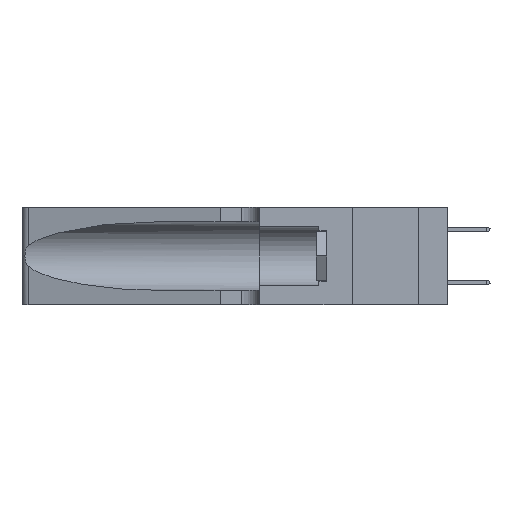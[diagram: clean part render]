
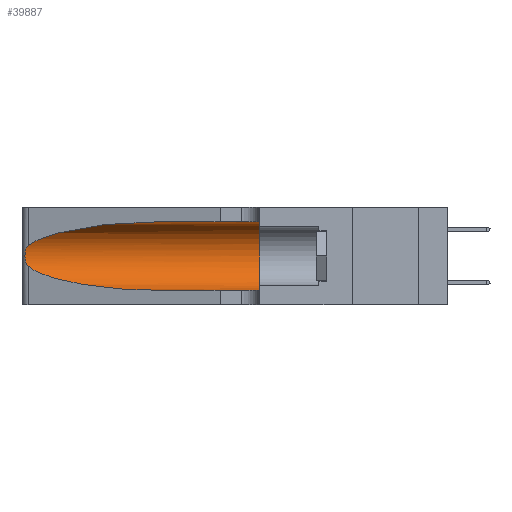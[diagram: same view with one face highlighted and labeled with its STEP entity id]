
A CAD part, left-side view. The second image highlights one B-rep face of the part: STEP entity #39887.
In plain terms, the highlighted cylindrical face has radius 3.308 mm (diameter 6.617 mm), a partial arc.
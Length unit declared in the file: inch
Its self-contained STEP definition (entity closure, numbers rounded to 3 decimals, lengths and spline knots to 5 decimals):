
#478 = CARTESIAN_POINT ( 'NONE',  ( 0.18966, 0.96281, 0.31525 ) ) ;
#2114 = CARTESIAN_POINT ( 'NONE',  ( 0.25487, 1.22718, 0.22369 ) ) ;
#2186 = CYLINDRICAL_SURFACE ( 'NONE', #13376, 0.13025 ) ;
#2251 = CARTESIAN_POINT ( 'NONE',  ( 0.26075, 1.23896, 0.19203 ) ) ;
#3133 = VERTEX_POINT ( 'NONE', #14538 ) ;
#3681 = CARTESIAN_POINT ( 'NONE',  ( 0.2373, 1.15595, 0.28018 ) ) ;
#5518 = CARTESIAN_POINT ( 'NONE',  ( 0.26017, 1.23833, 0.17102 ) ) ;
#5655 = CARTESIAN_POINT ( 'NONE',  ( 0.18966, 0.96281, 0.05475 ) ) ;
#7068 = VECTOR ( 'NONE', #11288, 39.37008 ) ;
#8756 = CARTESIAN_POINT ( 'NONE',  ( 0.25789, 1.23486, 0.15765 ) ) ;
#9062 = DIRECTION ( 'NONE',  ( 0., 1., 0. ) ) ;
#10516 = EDGE_CURVE ( 'NONE', #3133, #27288, #33962, .T. ) ;
#10904 = CARTESIAN_POINT ( 'NONE',  ( 0.1305, 0.35, 0.05475 ) ) ;
#11197 = EDGE_CURVE ( 'NONE', #15068, #31761, #40780, .T. ) ;
#11288 = DIRECTION ( 'NONE',  ( 0., -1., 0. ) ) ;
#11788 = CARTESIAN_POINT ( 'NONE',  ( 0.1305, 0.72297, 0.31525 ) ) ;
#11969 = CARTESIAN_POINT ( 'NONE',  ( 0.25555, 1.22993, 0.14849 ) ) ;
#11972 = CARTESIAN_POINT ( 'NONE',  ( 0.2373, 1.15595, 0.08982 ) ) ;
#12216 = EDGE_CURVE ( 'NONE', #15068, #3133, #19265, .T. ) ;
#12989 = CARTESIAN_POINT ( 'NONE',  ( 0.1305, 0.72297, 0.05475 ) ) ;
#13003 = CARTESIAN_POINT ( 'NONE',  ( 0.1305, 0.35, 0.31525 ) ) ;
#13142 = ORIENTED_EDGE ( 'NONE', *, *, #12216, .T. ) ;
#13376 = AXIS2_PLACEMENT_3D ( 'NONE', #39045, #26362, #20112 ) ;
#13377 = CIRCLE ( 'NONE', #17214, 0.13025 ) ;
#14538 = CARTESIAN_POINT ( 'NONE',  ( 0.25487, 1.22718, 0.22369 ) ) ;
#14853 = DIRECTION ( 'NONE',  ( 0., -1., 0. ) ) ;
#15068 = VERTEX_POINT ( 'NONE', #11788 ) ;
#15341 = ORIENTED_EDGE ( 'NONE', *, *, #11197, .F. ) ;
#15547 = VECTOR ( 'NONE', #14853, 39.37008 ) ;
#17214 = AXIS2_PLACEMENT_3D ( 'NONE', #28076, #9062, #31283 ) ;
#18062 = CARTESIAN_POINT ( 'NONE',  ( 0.1305, 1.61858, 0.31525 ) ) ;
#18241 = CARTESIAN_POINT ( 'NONE',  ( 0.25787, 1.23484, 0.2124 ) ) ;
#18343 = EDGE_CURVE ( 'NONE', #28424, #33393, #22978, .T. ) ;
#19232 = FACE_OUTER_BOUND ( 'NONE', #20370, .T. ) ;
#19265 =( BOUNDED_CURVE ( )  B_SPLINE_CURVE ( 3, ( #19623, #478, #3681, #26017 ),
 .UNSPECIFIED., .F., .F. ) 
 B_SPLINE_CURVE_WITH_KNOTS ( ( 4, 4 ),
 ( 1.5708, 2.84003 ),
 .UNSPECIFIED. ) 
 CURVE ( )  GEOMETRIC_REPRESENTATION_ITEM ( )  RATIONAL_B_SPLINE_CURVE ( ( 1., 0.87, 0.87, 1. ) ) 
 REPRESENTATION_ITEM ( '' )  );
#19623 = CARTESIAN_POINT ( 'NONE',  ( 0.1305, 0.72297, 0.31525 ) ) ;
#20112 = DIRECTION ( 'NONE',  ( 0., 0., -1. ) ) ;
#20370 = EDGE_LOOP ( 'NONE', ( #13142, #20879, #39255, #40070, #24231, #15341 ) ) ;
#20879 = ORIENTED_EDGE ( 'NONE', *, *, #10516, .T. ) ;
#21259 = EDGE_CURVE ( 'NONE', #31761, #33393, #13377, .T. ) ;
#21404 = CARTESIAN_POINT ( 'NONE',  ( 0.26018, 1.23835, 0.19895 ) ) ;
#22978 = LINE ( 'NONE', #30289, #7068 ) ;
#23589 =( BOUNDED_CURVE ( )  B_SPLINE_CURVE ( 3, ( #34126, #11972, #5655, #27910 ),
 .UNSPECIFIED., .F., .F. ) 
 B_SPLINE_CURVE_WITH_KNOTS ( ( 4, 4 ),
 ( 3.44316, 4.71239 ),
 .UNSPECIFIED. ) 
 CURVE ( )  GEOMETRIC_REPRESENTATION_ITEM ( )  RATIONAL_B_SPLINE_CURVE ( ( 1., 0.87, 0.87, 1. ) ) 
 REPRESENTATION_ITEM ( '' )  );
#24231 = ORIENTED_EDGE ( 'NONE', *, *, #21259, .F. ) ;
#24586 = CARTESIAN_POINT ( 'NONE',  ( 0.26075, 1.23896, 0.178 ) ) ;
#26017 = CARTESIAN_POINT ( 'NONE',  ( 0.25487, 1.22718, 0.22369 ) ) ;
#26362 = DIRECTION ( 'NONE',  ( 0., -1., 0. ) ) ;
#27288 = VERTEX_POINT ( 'NONE', #39952 ) ;
#27779 = CARTESIAN_POINT ( 'NONE',  ( 0.25856, 1.23593, 0.16098 ) ) ;
#27910 = CARTESIAN_POINT ( 'NONE',  ( 0.1305, 0.72297, 0.05475 ) ) ;
#28076 = CARTESIAN_POINT ( 'NONE',  ( 0.1305, 0.35, 0.185 ) ) ;
#28424 = VERTEX_POINT ( 'NONE', #12989 ) ;
#30289 = CARTESIAN_POINT ( 'NONE',  ( 0.1305, 1.61858, 0.05475 ) ) ;
#30814 = EDGE_CURVE ( 'NONE', #27288, #28424, #23589, .T. ) ;
#30972 = CARTESIAN_POINT ( 'NONE',  ( 0.25639, 1.23186, 0.15144 ) ) ;
#31283 = DIRECTION ( 'NONE',  ( 0., 0., 1. ) ) ;
#31761 = VERTEX_POINT ( 'NONE', #13003 ) ;
#33393 = VERTEX_POINT ( 'NONE', #10904 ) ;
#33962 = B_SPLINE_CURVE_WITH_KNOTS ( 'NONE', 3,
 ( #2114, #40208, #37137, #18241, #40342, #21404, #2251, #24586, #5518, #27779, #8756, #30972, #11969, #34124 ),
 .UNSPECIFIED., .F., .F.,
 ( 4, 2, 2, 2, 2, 2, 4 ),
 ( 0., 0.00027, 0.00053, 0.00107, 0.0016, 0.00187, 0.00214 ),
 .UNSPECIFIED. ) ;
#34124 = CARTESIAN_POINT ( 'NONE',  ( 0.25487, 1.22718, 0.14631 ) ) ;
#34126 = CARTESIAN_POINT ( 'NONE',  ( 0.25487, 1.22718, 0.14631 ) ) ;
#37137 = CARTESIAN_POINT ( 'NONE',  ( 0.25639, 1.23184, 0.21858 ) ) ;
#39045 = CARTESIAN_POINT ( 'NONE',  ( 0.1305, 1.61858, 0.185 ) ) ;
#39255 = ORIENTED_EDGE ( 'NONE', *, *, #30814, .T. ) ;
#39887 = ADVANCED_FACE ( 'NONE', ( #19232 ), #2186, .F. ) ;
#39952 = CARTESIAN_POINT ( 'NONE',  ( 0.25487, 1.22718, 0.14631 ) ) ;
#40070 = ORIENTED_EDGE ( 'NONE', *, *, #18343, .T. ) ;
#40208 = CARTESIAN_POINT ( 'NONE',  ( 0.25555, 1.22994, 0.2215 ) ) ;
#40342 = CARTESIAN_POINT ( 'NONE',  ( 0.25854, 1.2359, 0.20912 ) ) ;
#40780 = LINE ( 'NONE', #18062, #15547 ) ;
